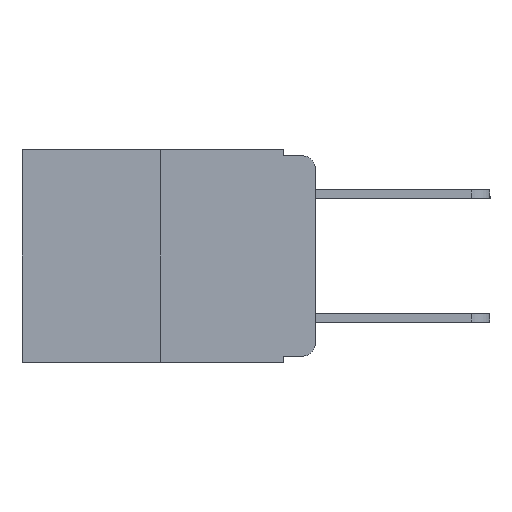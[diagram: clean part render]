
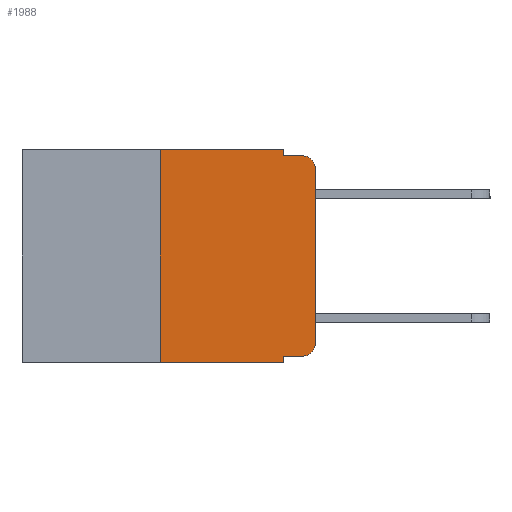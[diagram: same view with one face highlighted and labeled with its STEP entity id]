
A CAD part, left-side view. The second image highlights one B-rep face of the part: STEP entity #1988.
In plain terms, the highlighted planar face has unit normal (-1, 0, 0).
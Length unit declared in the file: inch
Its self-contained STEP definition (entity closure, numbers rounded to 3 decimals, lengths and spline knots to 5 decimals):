
#9 = AXIS2_PLACEMENT_3D ( 'NONE', #15334, #8983, #1339 ) ;
#141 = ORIENTED_EDGE ( 'NONE', *, *, #14292, .F. ) ;
#285 = DIRECTION ( 'NONE',  ( 0., -1., 0. ) ) ;
#298 = VERTEX_POINT ( 'NONE', #12294 ) ;
#354 = CARTESIAN_POINT ( 'NONE',  ( 0., 0.051, -0.333 ) ) ;
#365 = VERTEX_POINT ( 'NONE', #12327 ) ;
#566 = DIRECTION ( 'NONE',  ( 0., 0., 1. ) ) ;
#573 = CARTESIAN_POINT ( 'NONE',  ( 0., 0.473, -0.343 ) ) ;
#1077 = VECTOR ( 'NONE', #8090, 39.37008 ) ;
#1306 = FACE_OUTER_BOUND ( 'NONE', #5928, .T. ) ;
#1339 = DIRECTION ( 'NONE',  ( 0., 0., -1. ) ) ;
#1548 = VERTEX_POINT ( 'NONE', #12771 ) ;
#1872 = EDGE_CURVE ( 'NONE', #298, #1548, #13430, .T. ) ;
#1988 = ADVANCED_FACE ( 'NONE', ( #1306 ), #8954, .F. ) ;
#2057 = VERTEX_POINT ( 'NONE', #14127 ) ;
#2159 = ORIENTED_EDGE ( 'NONE', *, *, #1872, .F. ) ;
#2276 = VECTOR ( 'NONE', #15419, 39.37008 ) ;
#2514 = CARTESIAN_POINT ( 'NONE',  ( 0., 0.25, 0. ) ) ;
#2616 = DIRECTION ( 'NONE',  ( 0., -1., 0. ) ) ;
#3128 = CARTESIAN_POINT ( 'NONE',  ( 0., 0., -0.313 ) ) ;
#3202 = CARTESIAN_POINT ( 'NONE',  ( 0., 0.473, 0. ) ) ;
#3223 = VERTEX_POINT ( 'NONE', #3128 ) ;
#3330 = CIRCLE ( 'NONE', #6021, 0.02 ) ;
#3409 = VECTOR ( 'NONE', #566, 39.37008 ) ;
#3473 = VERTEX_POINT ( 'NONE', #14836 ) ;
#3482 = EDGE_CURVE ( 'NONE', #3223, #10870, #6708, .T. ) ;
#3912 = EDGE_CURVE ( 'NONE', #298, #365, #10336, .T. ) ;
#4367 = LINE ( 'NONE', #2514, #7548 ) ;
#4618 = VECTOR ( 'NONE', #8423, 39.37008 ) ;
#4636 = VECTOR ( 'NONE', #2616, 39.37008 ) ;
#5809 = LINE ( 'NONE', #10081, #2276 ) ;
#5833 = EDGE_CURVE ( 'NONE', #13160, #7766, #4367, .T. ) ;
#5928 = EDGE_LOOP ( 'NONE', ( #8258, #11223, #9825, #13204, #141, #9127, #11994, #2159, #7549, #7172 ) ) ;
#6021 = AXIS2_PLACEMENT_3D ( 'NONE', #6807, #14399, #7925 ) ;
#6155 = CARTESIAN_POINT ( 'NONE',  ( 0., 0.25, 0. ) ) ;
#6337 = CIRCLE ( 'NONE', #9, 0.02 ) ;
#6708 = LINE ( 'NONE', #14916, #3409 ) ;
#6807 = CARTESIAN_POINT ( 'NONE',  ( 0., 0.02, -0.313 ) ) ;
#7164 = VERTEX_POINT ( 'NONE', #14071 ) ;
#7172 = ORIENTED_EDGE ( 'NONE', *, *, #7263, .T. ) ;
#7251 = CARTESIAN_POINT ( 'NONE',  ( 0., 0.25, -0.343 ) ) ;
#7263 = EDGE_CURVE ( 'NONE', #365, #3223, #3330, .T. ) ;
#7548 = VECTOR ( 'NONE', #10802, 39.37008 ) ;
#7549 = ORIENTED_EDGE ( 'NONE', *, *, #3912, .T. ) ;
#7766 = VERTEX_POINT ( 'NONE', #6155 ) ;
#7780 = LINE ( 'NONE', #12998, #4636 ) ;
#7925 = DIRECTION ( 'NONE',  ( 0., 0., -1. ) ) ;
#8090 = DIRECTION ( 'NONE',  ( 0., 0., -1. ) ) ;
#8258 = ORIENTED_EDGE ( 'NONE', *, *, #3482, .T. ) ;
#8423 = DIRECTION ( 'NONE',  ( 0., -1., 0. ) ) ;
#8954 = PLANE ( 'NONE',  #13844 ) ;
#8983 = DIRECTION ( 'NONE',  ( -1., 0., 0. ) ) ;
#9127 = ORIENTED_EDGE ( 'NONE', *, *, #5833, .F. ) ;
#9825 = ORIENTED_EDGE ( 'NONE', *, *, #12221, .F. ) ;
#9982 = VECTOR ( 'NONE', #285, 39.37008 ) ;
#9983 = LINE ( 'NONE', #13806, #15315 ) ;
#10081 = CARTESIAN_POINT ( 'NONE',  ( 0., 0.473, 0. ) ) ;
#10150 = CARTESIAN_POINT ( 'NONE',  ( 0., 0.051, 0. ) ) ;
#10336 = LINE ( 'NONE', #354, #9982 ) ;
#10338 = LINE ( 'NONE', #573, #4618 ) ;
#10587 = DIRECTION ( 'NONE',  ( 0., 0., -1. ) ) ;
#10700 = CARTESIAN_POINT ( 'NONE',  ( 0., 0., -0.03 ) ) ;
#10802 = DIRECTION ( 'NONE',  ( 0., 0., 1. ) ) ;
#10870 = VERTEX_POINT ( 'NONE', #10700 ) ;
#11223 = ORIENTED_EDGE ( 'NONE', *, *, #12371, .T. ) ;
#11994 = ORIENTED_EDGE ( 'NONE', *, *, #12631, .T. ) ;
#12221 = EDGE_CURVE ( 'NONE', #2057, #7164, #7780, .T. ) ;
#12294 = CARTESIAN_POINT ( 'NONE',  ( 0., 0.051, -0.333 ) ) ;
#12327 = CARTESIAN_POINT ( 'NONE',  ( 0., 0.02, -0.333 ) ) ;
#12371 = EDGE_CURVE ( 'NONE', #10870, #7164, #6337, .T. ) ;
#12631 = EDGE_CURVE ( 'NONE', #13160, #1548, #10338, .T. ) ;
#12634 = EDGE_CURVE ( 'NONE', #3473, #2057, #9983, .T. ) ;
#12771 = CARTESIAN_POINT ( 'NONE',  ( 0., 0.051, -0.343 ) ) ;
#12998 = CARTESIAN_POINT ( 'NONE',  ( 0., 0.051, -0.01 ) ) ;
#13160 = VERTEX_POINT ( 'NONE', #7251 ) ;
#13204 = ORIENTED_EDGE ( 'NONE', *, *, #12634, .F. ) ;
#13430 = LINE ( 'NONE', #10150, #1077 ) ;
#13580 = DIRECTION ( 'NONE',  ( 1., 0., 0. ) ) ;
#13806 = CARTESIAN_POINT ( 'NONE',  ( 0., 0.051, 0. ) ) ;
#13844 = AXIS2_PLACEMENT_3D ( 'NONE', #3202, #13580, #10587 ) ;
#14071 = CARTESIAN_POINT ( 'NONE',  ( 0., 0.02, -0.01 ) ) ;
#14127 = CARTESIAN_POINT ( 'NONE',  ( 0., 0.051, -0.01 ) ) ;
#14292 = EDGE_CURVE ( 'NONE', #7766, #3473, #5809, .T. ) ;
#14399 = DIRECTION ( 'NONE',  ( -1., 0., 0. ) ) ;
#14836 = CARTESIAN_POINT ( 'NONE',  ( 0., 0.051, 0. ) ) ;
#14875 = DIRECTION ( 'NONE',  ( 0., 0., -1. ) ) ;
#14916 = CARTESIAN_POINT ( 'NONE',  ( 0., 0., 0. ) ) ;
#15315 = VECTOR ( 'NONE', #14875, 39.37008 ) ;
#15334 = CARTESIAN_POINT ( 'NONE',  ( 0., 0.02, -0.03 ) ) ;
#15419 = DIRECTION ( 'NONE',  ( 0., -1., 0. ) ) ;
